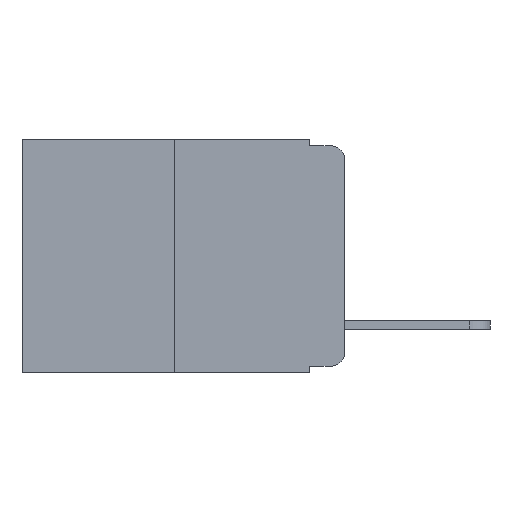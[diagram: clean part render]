
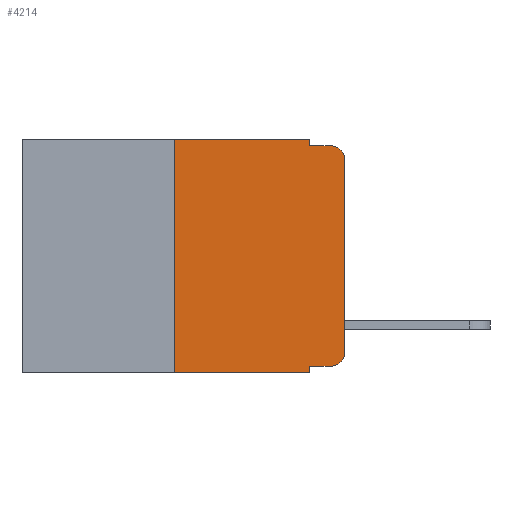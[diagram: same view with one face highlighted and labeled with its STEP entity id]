
A CAD part, left-side view. The second image highlights one B-rep face of the part: STEP entity #4214.
In plain terms, the highlighted planar face has unit normal (-1, 0, 0).
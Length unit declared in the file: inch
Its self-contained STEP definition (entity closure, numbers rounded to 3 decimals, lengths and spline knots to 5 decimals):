
#267 = ORIENTED_EDGE ( 'NONE', *, *, #6089, .T. ) ;
#357 = DIRECTION ( 'NONE',  ( 0., -1., 0. ) ) ;
#965 = ORIENTED_EDGE ( 'NONE', *, *, #6163, .F. ) ;
#1171 = VERTEX_POINT ( 'NONE', #11363 ) ;
#1203 = EDGE_CURVE ( 'NONE', #18856, #9663, #16633, .T. ) ;
#1276 = VECTOR ( 'NONE', #4031, 39.37008 ) ;
#1589 = VERTEX_POINT ( 'NONE', #12691 ) ;
#1684 = ORIENTED_EDGE ( 'NONE', *, *, #6408, .F. ) ;
#1689 = VERTEX_POINT ( 'NONE', #2758 ) ;
#1792 = CARTESIAN_POINT ( 'NONE',  ( 0., 0.051, -0.01 ) ) ;
#1994 = VERTEX_POINT ( 'NONE', #18831 ) ;
#2026 = LINE ( 'NONE', #4053, #1276 ) ;
#2758 = CARTESIAN_POINT ( 'NONE',  ( 0., 0., -0.313 ) ) ;
#3810 = AXIS2_PLACEMENT_3D ( 'NONE', #6423, #5539, #5171 ) ;
#3921 = VERTEX_POINT ( 'NONE', #10785 ) ;
#4031 = DIRECTION ( 'NONE',  ( 0., 0., 1. ) ) ;
#4053 = CARTESIAN_POINT ( 'NONE',  ( 0., 0., 0. ) ) ;
#4152 = DIRECTION ( 'NONE',  ( 0., 0., -1. ) ) ;
#4157 = DIRECTION ( 'NONE',  ( -1., 0., 0. ) ) ;
#4188 = CARTESIAN_POINT ( 'NONE',  ( 0., 0.02, -0.03 ) ) ;
#4214 = ADVANCED_FACE ( 'NONE', ( #5803 ), #5931, .F. ) ;
#4575 = CARTESIAN_POINT ( 'NONE',  ( 0., 0.473, 0. ) ) ;
#4712 = DIRECTION ( 'NONE',  ( 0., -1., 0. ) ) ;
#4715 = CARTESIAN_POINT ( 'NONE',  ( 0., 0.051, -0.01 ) ) ;
#4871 = LINE ( 'NONE', #6075, #9289 ) ;
#5171 = DIRECTION ( 'NONE',  ( 0., 0., -1. ) ) ;
#5242 = ORIENTED_EDGE ( 'NONE', *, *, #6236, .F. ) ;
#5539 = DIRECTION ( 'NONE',  ( 1., 0., 0. ) ) ;
#5803 = FACE_OUTER_BOUND ( 'NONE', #8242, .T. ) ;
#5931 = PLANE ( 'NONE',  #3810 ) ;
#6030 = DIRECTION ( 'NONE',  ( 0., 0., -1. ) ) ;
#6075 = CARTESIAN_POINT ( 'NONE',  ( 0., 0.051, 0. ) ) ;
#6089 = EDGE_CURVE ( 'NONE', #1994, #1689, #12179, .T. ) ;
#6101 = VECTOR ( 'NONE', #7028, 39.37008 ) ;
#6122 = EDGE_CURVE ( 'NONE', #1171, #1994, #16197, .T. ) ;
#6163 = EDGE_CURVE ( 'NONE', #1171, #1589, #11062, .T. ) ;
#6235 = EDGE_CURVE ( 'NONE', #11661, #18856, #9908, .T. ) ;
#6236 = EDGE_CURVE ( 'NONE', #9663, #12700, #4871, .T. ) ;
#6338 = DIRECTION ( 'NONE',  ( 0., 0., 1. ) ) ;
#6408 = EDGE_CURVE ( 'NONE', #12700, #3921, #17046, .T. ) ;
#6423 = CARTESIAN_POINT ( 'NONE',  ( 0., 0.473, 0. ) ) ;
#6449 = EDGE_CURVE ( 'NONE', #11699, #3921, #21060, .T. ) ;
#6479 = EDGE_CURVE ( 'NONE', #1689, #11699, #2026, .T. ) ;
#6544 = CARTESIAN_POINT ( 'NONE',  ( 0., 0.25, 0. ) ) ;
#6588 = CARTESIAN_POINT ( 'NONE',  ( 0., 0.25, 0. ) ) ;
#7028 = DIRECTION ( 'NONE',  ( 0., 0., -1. ) ) ;
#7043 = AXIS2_PLACEMENT_3D ( 'NONE', #7864, #7839, #7790 ) ;
#7216 = CARTESIAN_POINT ( 'NONE',  ( 0., 0.051, 0. ) ) ;
#7641 = DIRECTION ( 'NONE',  ( 0., -1., 0. ) ) ;
#7698 = CARTESIAN_POINT ( 'NONE',  ( 0., 0.051, -0.333 ) ) ;
#7769 = VECTOR ( 'NONE', #357, 39.37008 ) ;
#7790 = DIRECTION ( 'NONE',  ( 0., 0., -1. ) ) ;
#7839 = DIRECTION ( 'NONE',  ( -1., 0., 0. ) ) ;
#7864 = CARTESIAN_POINT ( 'NONE',  ( 0., 0.02, -0.313 ) ) ;
#8178 = VECTOR ( 'NONE', #4712, 39.37008 ) ;
#8242 = EDGE_LOOP ( 'NONE', ( #13677, #20047, #1684, #5242, #12674, #22032, #13766, #965, #19345, #267 ) ) ;
#9041 = AXIS2_PLACEMENT_3D ( 'NONE', #4188, #4157, #4152 ) ;
#9289 = VECTOR ( 'NONE', #6030, 39.37008 ) ;
#9615 = VECTOR ( 'NONE', #12000, 39.37008 ) ;
#9663 = VERTEX_POINT ( 'NONE', #17279 ) ;
#9908 = LINE ( 'NONE', #6544, #15039 ) ;
#10785 = CARTESIAN_POINT ( 'NONE',  ( 0., 0.02, -0.01 ) ) ;
#11062 = LINE ( 'NONE', #7216, #6101 ) ;
#11363 = CARTESIAN_POINT ( 'NONE',  ( 0., 0.051, -0.333 ) ) ;
#11661 = VERTEX_POINT ( 'NONE', #18844 ) ;
#11699 = VERTEX_POINT ( 'NONE', #18768 ) ;
#12000 = DIRECTION ( 'NONE',  ( 0., -1., 0. ) ) ;
#12179 = CIRCLE ( 'NONE', #7043, 0.02 ) ;
#12674 = ORIENTED_EDGE ( 'NONE', *, *, #1203, .F. ) ;
#12691 = CARTESIAN_POINT ( 'NONE',  ( 0., 0.051, -0.343 ) ) ;
#12700 = VERTEX_POINT ( 'NONE', #1792 ) ;
#13675 = CARTESIAN_POINT ( 'NONE',  ( 0., 0.473, -0.343 ) ) ;
#13677 = ORIENTED_EDGE ( 'NONE', *, *, #6479, .T. ) ;
#13766 = ORIENTED_EDGE ( 'NONE', *, *, #22797, .T. ) ;
#15039 = VECTOR ( 'NONE', #6338, 39.37008 ) ;
#16197 = LINE ( 'NONE', #7698, #20802 ) ;
#16633 = LINE ( 'NONE', #4575, #7769 ) ;
#17046 = LINE ( 'NONE', #4715, #8178 ) ;
#17279 = CARTESIAN_POINT ( 'NONE',  ( 0., 0.051, 0. ) ) ;
#18768 = CARTESIAN_POINT ( 'NONE',  ( 0., 0., -0.03 ) ) ;
#18831 = CARTESIAN_POINT ( 'NONE',  ( 0., 0.02, -0.333 ) ) ;
#18844 = CARTESIAN_POINT ( 'NONE',  ( 0., 0.25, -0.343 ) ) ;
#18856 = VERTEX_POINT ( 'NONE', #6588 ) ;
#19345 = ORIENTED_EDGE ( 'NONE', *, *, #6122, .T. ) ;
#20047 = ORIENTED_EDGE ( 'NONE', *, *, #6449, .T. ) ;
#20802 = VECTOR ( 'NONE', #7641, 39.37008 ) ;
#21060 = CIRCLE ( 'NONE', #9041, 0.02 ) ;
#22032 = ORIENTED_EDGE ( 'NONE', *, *, #6235, .F. ) ;
#22797 = EDGE_CURVE ( 'NONE', #11661, #1589, #23412, .T. ) ;
#23412 = LINE ( 'NONE', #13675, #9615 ) ;
